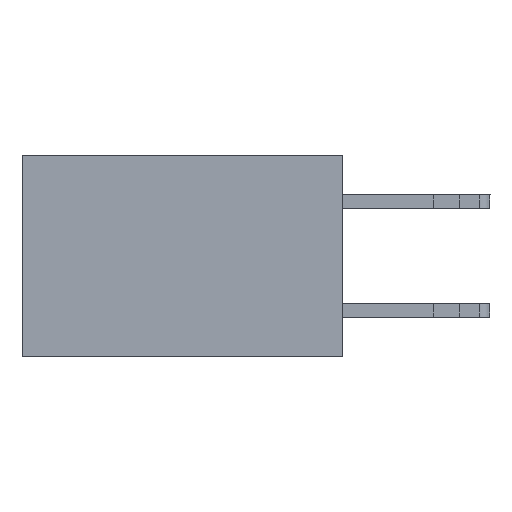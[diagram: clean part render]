
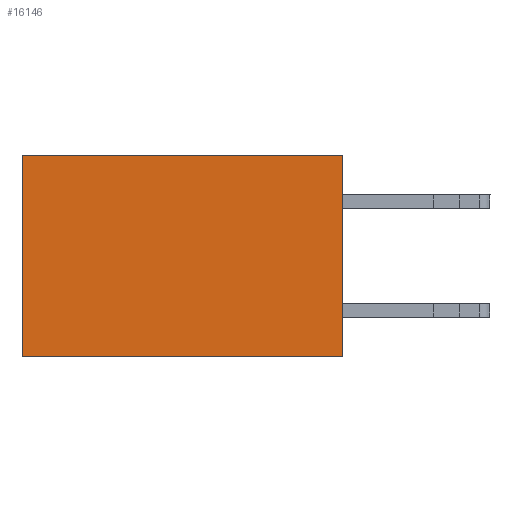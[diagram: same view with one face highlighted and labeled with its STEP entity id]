
A CAD part, left-side view. The second image highlights one B-rep face of the part: STEP entity #16146.
In plain terms, the highlighted planar face has unit normal (-1, 0, 0).
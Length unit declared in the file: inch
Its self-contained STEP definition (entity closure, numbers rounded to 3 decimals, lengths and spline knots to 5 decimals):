
#75 = VERTEX_POINT ( 'NONE', #3456 ) ;
#219 = EDGE_CURVE ( 'NONE', #18782, #11053, #1953, .T. ) ;
#908 = DIRECTION ( 'NONE',  ( 0., 0., -1. ) ) ;
#1106 = AXIS2_PLACEMENT_3D ( 'NONE', #22860, #21370, #4215 ) ;
#1735 = CARTESIAN_POINT ( 'NONE',  ( 0.277, 0., -0.37 ) ) ;
#1852 = EDGE_CURVE ( 'NONE', #75, #7331, #22577, .T. ) ;
#1953 = LINE ( 'NONE', #11416, #13180 ) ;
#1970 = CARTESIAN_POINT ( 'NONE',  ( 0.277, 0., -0.37 ) ) ;
#2763 = LINE ( 'NONE', #23646, #4410 ) ;
#3108 = ORIENTED_EDGE ( 'NONE', *, *, #219, .F. ) ;
#3456 = CARTESIAN_POINT ( 'NONE',  ( 0.277, 0., 0. ) ) ;
#4215 = DIRECTION ( 'NONE',  ( 0., 0., -1. ) ) ;
#4410 = VECTOR ( 'NONE', #908, 39.37008 ) ;
#7331 = VERTEX_POINT ( 'NONE', #13094 ) ;
#8235 = ORIENTED_EDGE ( 'NONE', *, *, #18100, .T. ) ;
#9551 = DIRECTION ( 'NONE',  ( 0., 0., -1. ) ) ;
#11053 = VERTEX_POINT ( 'NONE', #13725 ) ;
#11416 = CARTESIAN_POINT ( 'NONE',  ( 0.277, 0., -0.37 ) ) ;
#11673 = VECTOR ( 'NONE', #9551, 39.37008 ) ;
#13094 = CARTESIAN_POINT ( 'NONE',  ( 0.277, 0.59, 0. ) ) ;
#13180 = VECTOR ( 'NONE', #17021, 39.37008 ) ;
#13725 = CARTESIAN_POINT ( 'NONE',  ( 0.277, 0.59, -0.37 ) ) ;
#14849 = VECTOR ( 'NONE', #22334, 39.37008 ) ;
#15303 = ORIENTED_EDGE ( 'NONE', *, *, #1852, .T. ) ;
#15312 = FACE_OUTER_BOUND ( 'NONE', #16844, .T. ) ;
#16146 = ADVANCED_FACE ( 'NONE', ( #15312 ), #19527, .F. ) ;
#16844 = EDGE_LOOP ( 'NONE', ( #8235, #3108, #21998, #15303 ) ) ;
#17021 = DIRECTION ( 'NONE',  ( 0., 1., 0. ) ) ;
#18100 = EDGE_CURVE ( 'NONE', #7331, #11053, #2763, .T. ) ;
#18782 = VERTEX_POINT ( 'NONE', #1735 ) ;
#19285 = LINE ( 'NONE', #1970, #11673 ) ;
#19527 = PLANE ( 'NONE',  #1106 ) ;
#20370 = CARTESIAN_POINT ( 'NONE',  ( 0.277, 0., 0. ) ) ;
#21370 = DIRECTION ( 'NONE',  ( 1., 0., 0. ) ) ;
#21998 = ORIENTED_EDGE ( 'NONE', *, *, #22918, .F. ) ;
#22334 = DIRECTION ( 'NONE',  ( 0., 1., 0. ) ) ;
#22577 = LINE ( 'NONE', #20370, #14849 ) ;
#22860 = CARTESIAN_POINT ( 'NONE',  ( 0.277, 0., -0.37 ) ) ;
#22918 = EDGE_CURVE ( 'NONE', #75, #18782, #19285, .T. ) ;
#23646 = CARTESIAN_POINT ( 'NONE',  ( 0.277, 0.59, -0.37 ) ) ;
